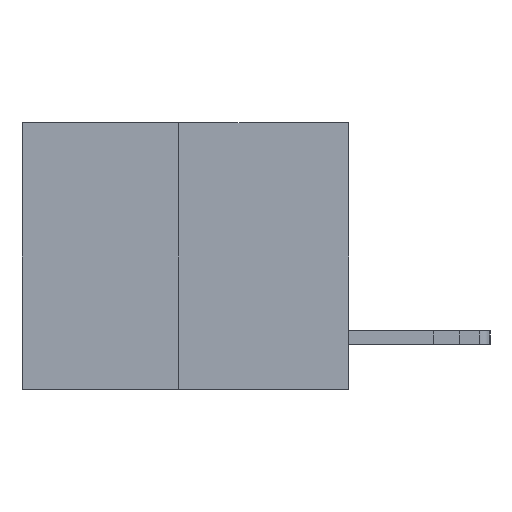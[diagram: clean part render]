
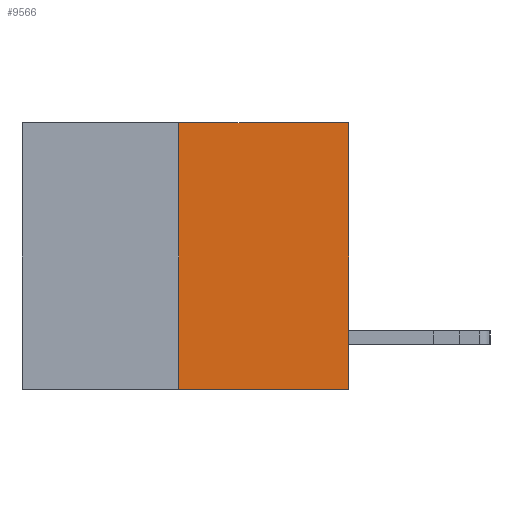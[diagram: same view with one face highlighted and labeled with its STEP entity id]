
A CAD part, left-side view. The second image highlights one B-rep face of the part: STEP entity #9566.
In plain terms, the highlighted planar face has unit normal (-1, 0, 0).
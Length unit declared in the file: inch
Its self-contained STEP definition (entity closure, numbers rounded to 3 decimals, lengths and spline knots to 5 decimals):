
#512 = VECTOR ( 'NONE', #2370, 39.37008 ) ;
#799 = EDGE_LOOP ( 'NONE', ( #21718, #7268, #18368, #13625 ) ) ;
#2370 = DIRECTION ( 'NONE',  ( 0., -1., 0. ) ) ;
#2883 = LINE ( 'NONE', #8730, #5986 ) ;
#3254 = EDGE_CURVE ( 'NONE', #7854, #18028, #4049, .T. ) ;
#3539 = EDGE_CURVE ( 'NONE', #18028, #17565, #9965, .T. ) ;
#4049 = LINE ( 'NONE', #4695, #19927 ) ;
#4695 = CARTESIAN_POINT ( 'NONE',  ( 0., 0.6, -0.49 ) ) ;
#5230 = DIRECTION ( 'NONE',  ( 0., 0., 1. ) ) ;
#5312 = LINE ( 'NONE', #6017, #512 ) ;
#5476 = FACE_OUTER_BOUND ( 'NONE', #799, .T. ) ;
#5986 = VECTOR ( 'NONE', #12378, 39.37008 ) ;
#6017 = CARTESIAN_POINT ( 'NONE',  ( 0., 0.6, 0. ) ) ;
#7094 = PLANE ( 'NONE',  #12477 ) ;
#7218 = CARTESIAN_POINT ( 'NONE',  ( 0., 0.312, -0.49 ) ) ;
#7268 = ORIENTED_EDGE ( 'NONE', *, *, #3254, .T. ) ;
#7367 = CARTESIAN_POINT ( 'NONE',  ( 0., 0., -0.49 ) ) ;
#7854 = VERTEX_POINT ( 'NONE', #7218 ) ;
#8730 = CARTESIAN_POINT ( 'NONE',  ( 0., 0.312, -0.49 ) ) ;
#9566 = ADVANCED_FACE ( 'NONE', ( #5476 ), #7094, .F. ) ;
#9965 = LINE ( 'NONE', #10859, #18755 ) ;
#10163 = EDGE_CURVE ( 'NONE', #7854, #16477, #2883, .T. ) ;
#10859 = CARTESIAN_POINT ( 'NONE',  ( 0., 0., 0. ) ) ;
#12378 = DIRECTION ( 'NONE',  ( 0., 0., 1. ) ) ;
#12404 = CARTESIAN_POINT ( 'NONE',  ( 0., 0.6, 0. ) ) ;
#12477 = AXIS2_PLACEMENT_3D ( 'NONE', #12404, #14381, #23133 ) ;
#13625 = ORIENTED_EDGE ( 'NONE', *, *, #15800, .F. ) ;
#14381 = DIRECTION ( 'NONE',  ( 1., 0., 0. ) ) ;
#15800 = EDGE_CURVE ( 'NONE', #16477, #17565, #5312, .T. ) ;
#16477 = VERTEX_POINT ( 'NONE', #20295 ) ;
#17212 = CARTESIAN_POINT ( 'NONE',  ( 0., 0., 0. ) ) ;
#17565 = VERTEX_POINT ( 'NONE', #17212 ) ;
#18028 = VERTEX_POINT ( 'NONE', #7367 ) ;
#18368 = ORIENTED_EDGE ( 'NONE', *, *, #3539, .T. ) ;
#18755 = VECTOR ( 'NONE', #5230, 39.37008 ) ;
#19927 = VECTOR ( 'NONE', #21109, 39.37008 ) ;
#20295 = CARTESIAN_POINT ( 'NONE',  ( 0., 0.312, 0. ) ) ;
#21109 = DIRECTION ( 'NONE',  ( 0., -1., 0. ) ) ;
#21718 = ORIENTED_EDGE ( 'NONE', *, *, #10163, .F. ) ;
#23133 = DIRECTION ( 'NONE',  ( 0., 0., -1. ) ) ;
